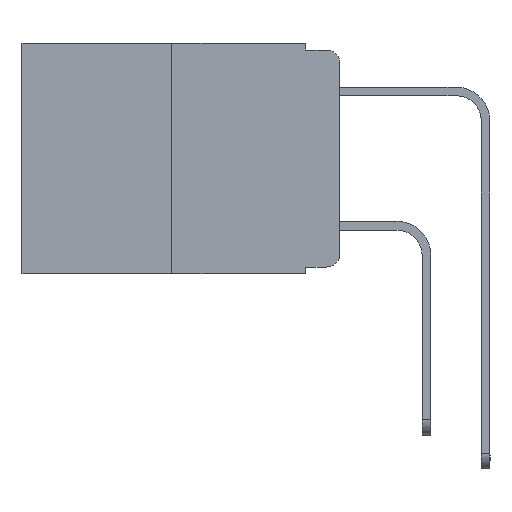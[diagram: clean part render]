
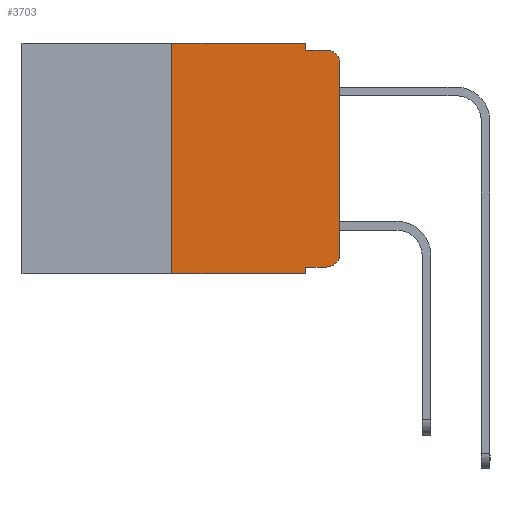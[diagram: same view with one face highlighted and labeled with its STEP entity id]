
A CAD part, left-side view. The second image highlights one B-rep face of the part: STEP entity #3703.
In plain terms, the highlighted planar face has unit normal (-1, 0, 0).
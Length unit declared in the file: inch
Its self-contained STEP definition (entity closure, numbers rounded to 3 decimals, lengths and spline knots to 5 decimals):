
#119 = CARTESIAN_POINT ( 'NONE',  ( 0., 0.473, 0. ) ) ;
#191 = EDGE_CURVE ( 'NONE', #21154, #6292, #17270, .T. ) ;
#627 = DIRECTION ( 'NONE',  ( 0., -1., 0. ) ) ;
#741 = LINE ( 'NONE', #11389, #16880 ) ;
#1019 = VECTOR ( 'NONE', #22194, 39.37008 ) ;
#1307 = VECTOR ( 'NONE', #5558, 39.37008 ) ;
#1361 = VERTEX_POINT ( 'NONE', #2013 ) ;
#1677 = VECTOR ( 'NONE', #8808, 39.37008 ) ;
#1913 = VERTEX_POINT ( 'NONE', #9683 ) ;
#2013 = CARTESIAN_POINT ( 'NONE',  ( 0., 0.02, -0.01 ) ) ;
#2030 = LINE ( 'NONE', #12250, #1307 ) ;
#2297 = VERTEX_POINT ( 'NONE', #8059 ) ;
#2609 = LINE ( 'NONE', #9755, #22065 ) ;
#3051 = EDGE_CURVE ( 'NONE', #9965, #1361, #741, .T. ) ;
#3278 = ORIENTED_EDGE ( 'NONE', *, *, #191, .T. ) ;
#3420 = EDGE_CURVE ( 'NONE', #1913, #2297, #8166, .T. ) ;
#3531 = DIRECTION ( 'NONE',  ( 0., 0., -1. ) ) ;
#3703 = ADVANCED_FACE ( 'NONE', ( #20952 ), #15422, .F. ) ;
#3825 = CIRCLE ( 'NONE', #12859, 0.02 ) ;
#4107 = CARTESIAN_POINT ( 'NONE',  ( 0., 0.051, -0.01 ) ) ;
#4210 = DIRECTION ( 'NONE',  ( 0., -1., 0. ) ) ;
#4289 = CARTESIAN_POINT ( 'NONE',  ( 0., 0.051, 0. ) ) ;
#4391 = CARTESIAN_POINT ( 'NONE',  ( 0., 0.25, 0. ) ) ;
#4658 = VERTEX_POINT ( 'NONE', #15574 ) ;
#5006 = EDGE_CURVE ( 'NONE', #12850, #5637, #22331, .T. ) ;
#5113 = EDGE_CURVE ( 'NONE', #5637, #9965, #5466, .T. ) ;
#5346 = DIRECTION ( 'NONE',  ( 1., 0., 0. ) ) ;
#5452 = CARTESIAN_POINT ( 'NONE',  ( 0., 0.051, -0.333 ) ) ;
#5466 = LINE ( 'NONE', #10452, #6005 ) ;
#5558 = DIRECTION ( 'NONE',  ( 0., 0., 1. ) ) ;
#5637 = VERTEX_POINT ( 'NONE', #4289 ) ;
#6005 = VECTOR ( 'NONE', #19264, 39.37008 ) ;
#6198 = EDGE_CURVE ( 'NONE', #4658, #1361, #3825, .T. ) ;
#6292 = VERTEX_POINT ( 'NONE', #11827 ) ;
#6431 = AXIS2_PLACEMENT_3D ( 'NONE', #16716, #9818, #17050 ) ;
#6811 = EDGE_CURVE ( 'NONE', #6292, #4658, #2030, .T. ) ;
#8059 = CARTESIAN_POINT ( 'NONE',  ( 0., 0.051, -0.343 ) ) ;
#8060 = EDGE_LOOP ( 'NONE', ( #10757, #22090, #16782, #15971, #9001, #13940, #20101, #13195, #15255, #3278 ) ) ;
#8166 = LINE ( 'NONE', #8281, #1019 ) ;
#8281 = CARTESIAN_POINT ( 'NONE',  ( 0., 0.473, -0.343 ) ) ;
#8808 = DIRECTION ( 'NONE',  ( 0., 0., -1. ) ) ;
#9001 = ORIENTED_EDGE ( 'NONE', *, *, #5006, .F. ) ;
#9497 = DIRECTION ( 'NONE',  ( 0., 0., 1. ) ) ;
#9683 = CARTESIAN_POINT ( 'NONE',  ( 0., 0.25, -0.343 ) ) ;
#9755 = CARTESIAN_POINT ( 'NONE',  ( 0., 0.051, -0.333 ) ) ;
#9818 = DIRECTION ( 'NONE',  ( -1., 0., 0. ) ) ;
#9965 = VERTEX_POINT ( 'NONE', #4107 ) ;
#10452 = CARTESIAN_POINT ( 'NONE',  ( 0., 0.051, 0. ) ) ;
#10757 = ORIENTED_EDGE ( 'NONE', *, *, #6811, .T. ) ;
#11389 = CARTESIAN_POINT ( 'NONE',  ( 0., 0.051, -0.01 ) ) ;
#11512 = CARTESIAN_POINT ( 'NONE',  ( 0., 0.02, -0.333 ) ) ;
#11603 = CARTESIAN_POINT ( 'NONE',  ( 0., 0.02, -0.03 ) ) ;
#11710 = DIRECTION ( 'NONE',  ( -1., 0., 0. ) ) ;
#11827 = CARTESIAN_POINT ( 'NONE',  ( 0., 0., -0.313 ) ) ;
#12250 = CARTESIAN_POINT ( 'NONE',  ( 0., 0., 0. ) ) ;
#12850 = VERTEX_POINT ( 'NONE', #19627 ) ;
#12859 = AXIS2_PLACEMENT_3D ( 'NONE', #11603, #11710, #15208 ) ;
#13195 = ORIENTED_EDGE ( 'NONE', *, *, #22187, .F. ) ;
#13381 = EDGE_CURVE ( 'NONE', #14897, #21154, #2609, .T. ) ;
#13392 = CARTESIAN_POINT ( 'NONE',  ( 0., 0.473, 0. ) ) ;
#13940 = ORIENTED_EDGE ( 'NONE', *, *, #20499, .F. ) ;
#14340 = VECTOR ( 'NONE', #22098, 39.37008 ) ;
#14897 = VERTEX_POINT ( 'NONE', #5452 ) ;
#15208 = DIRECTION ( 'NONE',  ( 0., 0., -1. ) ) ;
#15255 = ORIENTED_EDGE ( 'NONE', *, *, #13381, .T. ) ;
#15422 = PLANE ( 'NONE',  #19321 ) ;
#15574 = CARTESIAN_POINT ( 'NONE',  ( 0., 0., -0.03 ) ) ;
#15971 = ORIENTED_EDGE ( 'NONE', *, *, #5113, .F. ) ;
#16716 = CARTESIAN_POINT ( 'NONE',  ( 0., 0.02, -0.313 ) ) ;
#16782 = ORIENTED_EDGE ( 'NONE', *, *, #3051, .F. ) ;
#16880 = VECTOR ( 'NONE', #627, 39.37008 ) ;
#17050 = DIRECTION ( 'NONE',  ( 0., 0., -1. ) ) ;
#17270 = CIRCLE ( 'NONE', #6431, 0.02 ) ;
#17864 = LINE ( 'NONE', #4391, #19712 ) ;
#19097 = CARTESIAN_POINT ( 'NONE',  ( 0., 0.051, 0. ) ) ;
#19264 = DIRECTION ( 'NONE',  ( 0., 0., -1. ) ) ;
#19321 = AXIS2_PLACEMENT_3D ( 'NONE', #119, #5346, #3531 ) ;
#19432 = LINE ( 'NONE', #19097, #1677 ) ;
#19627 = CARTESIAN_POINT ( 'NONE',  ( 0., 0.25, 0. ) ) ;
#19712 = VECTOR ( 'NONE', #9497, 39.37008 ) ;
#20101 = ORIENTED_EDGE ( 'NONE', *, *, #3420, .T. ) ;
#20499 = EDGE_CURVE ( 'NONE', #1913, #12850, #17864, .T. ) ;
#20952 = FACE_OUTER_BOUND ( 'NONE', #8060, .T. ) ;
#21154 = VERTEX_POINT ( 'NONE', #11512 ) ;
#22065 = VECTOR ( 'NONE', #4210, 39.37008 ) ;
#22090 = ORIENTED_EDGE ( 'NONE', *, *, #6198, .T. ) ;
#22098 = DIRECTION ( 'NONE',  ( 0., -1., 0. ) ) ;
#22187 = EDGE_CURVE ( 'NONE', #14897, #2297, #19432, .T. ) ;
#22194 = DIRECTION ( 'NONE',  ( 0., -1., 0. ) ) ;
#22331 = LINE ( 'NONE', #13392, #14340 ) ;
